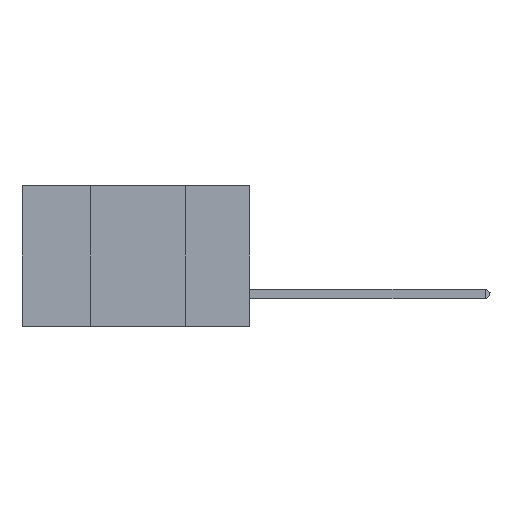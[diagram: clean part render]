
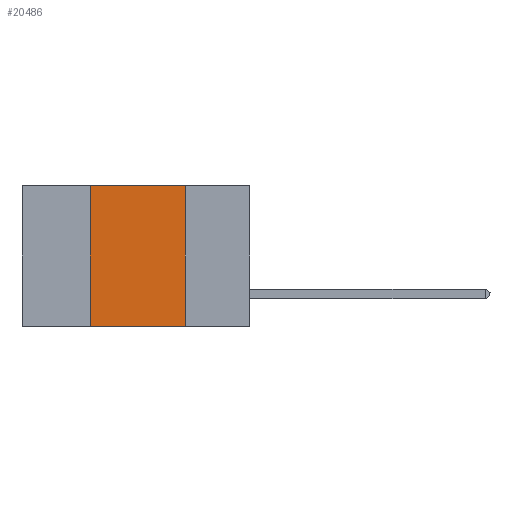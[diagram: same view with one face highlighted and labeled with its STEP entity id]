
A CAD part, left-side view. The second image highlights one B-rep face of the part: STEP entity #20486.
In plain terms, the highlighted planar face has unit normal (-1, 0, 0).
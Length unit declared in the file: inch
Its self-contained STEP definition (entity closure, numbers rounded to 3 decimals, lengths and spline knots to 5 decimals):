
#481 = CARTESIAN_POINT ( 'NONE',  ( 0., 0.17, 0. ) ) ;
#2288 = CARTESIAN_POINT ( 'NONE',  ( 0., 0.42, 0. ) ) ;
#2503 = DIRECTION ( 'NONE',  ( 1., 0., 0. ) ) ;
#2980 = DIRECTION ( 'NONE',  ( 0., -1., 0. ) ) ;
#4469 = ORIENTED_EDGE ( 'NONE', *, *, #9708, .F. ) ;
#5078 = CARTESIAN_POINT ( 'NONE',  ( 0., 0.42, -0.37 ) ) ;
#6435 = VERTEX_POINT ( 'NONE', #20986 ) ;
#9708 = EDGE_CURVE ( 'NONE', #28927, #6435, #29978, .T. ) ;
#10277 = DIRECTION ( 'NONE',  ( 0., 0., -1. ) ) ;
#11078 = CARTESIAN_POINT ( 'NONE',  ( 0., 0.17, 0. ) ) ;
#11267 = LINE ( 'NONE', #21675, #26621 ) ;
#13438 = CARTESIAN_POINT ( 'NONE',  ( 0., 0.6, 0. ) ) ;
#16500 = ORIENTED_EDGE ( 'NONE', *, *, #47212, .F. ) ;
#18480 = LINE ( 'NONE', #41824, #42714 ) ;
#18694 = EDGE_CURVE ( 'NONE', #43695, #6435, #11267, .T. ) ;
#20486 = ADVANCED_FACE ( 'NONE', ( #37050 ), #28614, .F. ) ;
#20986 = CARTESIAN_POINT ( 'NONE',  ( 0., 0.17, -0.37 ) ) ;
#21509 = CARTESIAN_POINT ( 'NONE',  ( 0., 0.6, 0. ) ) ;
#21675 = CARTESIAN_POINT ( 'NONE',  ( 0., 0.6, -0.37 ) ) ;
#23074 = LINE ( 'NONE', #13438, #40830 ) ;
#24617 = EDGE_CURVE ( 'NONE', #43695, #43785, #18480, .T. ) ;
#26621 = VECTOR ( 'NONE', #2980, 39.37008 ) ;
#28614 = PLANE ( 'NONE',  #35742 ) ;
#28927 = VERTEX_POINT ( 'NONE', #11078 ) ;
#29978 = LINE ( 'NONE', #481, #37669 ) ;
#30301 = ORIENTED_EDGE ( 'NONE', *, *, #18694, .T. ) ;
#34400 = DIRECTION ( 'NONE',  ( 0., 0., -1. ) ) ;
#35742 = AXIS2_PLACEMENT_3D ( 'NONE', #21509, #2503, #10277 ) ;
#36976 = EDGE_LOOP ( 'NONE', ( #4469, #16500, #39728, #30301 ) ) ;
#37050 = FACE_OUTER_BOUND ( 'NONE', #36976, .T. ) ;
#37669 = VECTOR ( 'NONE', #34400, 39.37008 ) ;
#39728 = ORIENTED_EDGE ( 'NONE', *, *, #24617, .F. ) ;
#40830 = VECTOR ( 'NONE', #47530, 39.37008 ) ;
#41824 = CARTESIAN_POINT ( 'NONE',  ( 0., 0.42, 0. ) ) ;
#42714 = VECTOR ( 'NONE', #46453, 39.37008 ) ;
#43695 = VERTEX_POINT ( 'NONE', #5078 ) ;
#43785 = VERTEX_POINT ( 'NONE', #2288 ) ;
#46453 = DIRECTION ( 'NONE',  ( 0., 0., 1. ) ) ;
#47212 = EDGE_CURVE ( 'NONE', #43785, #28927, #23074, .T. ) ;
#47530 = DIRECTION ( 'NONE',  ( 0., -1., 0. ) ) ;
